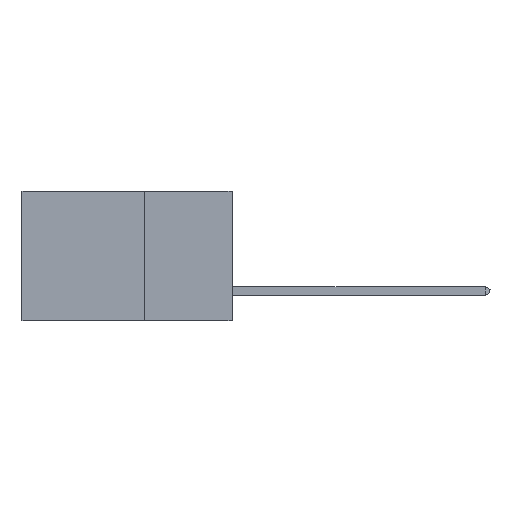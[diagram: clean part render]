
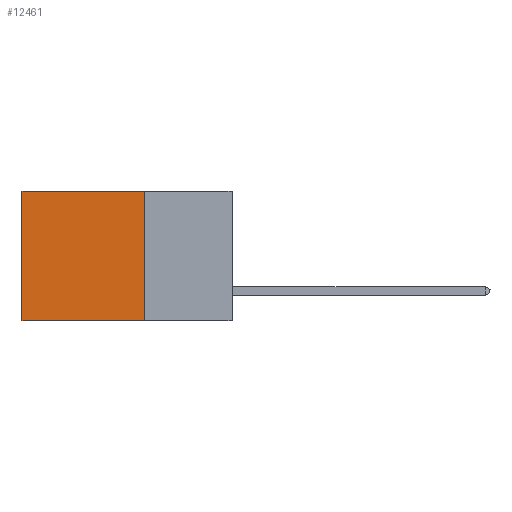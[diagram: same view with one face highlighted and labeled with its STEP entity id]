
A CAD part, left-side view. The second image highlights one B-rep face of the part: STEP entity #12461.
In plain terms, the highlighted planar face has unit normal (-1, 0, 0).
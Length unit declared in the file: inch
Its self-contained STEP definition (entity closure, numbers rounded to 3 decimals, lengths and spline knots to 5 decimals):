
#903 = EDGE_CURVE ( 'NONE', #23160, #5091, #25538, .T. ) ;
#1107 = EDGE_CURVE ( 'NONE', #5091, #11300, #23651, .T. ) ;
#1490 = DIRECTION ( 'NONE',  ( 0., 0., -1. ) ) ;
#1518 = EDGE_CURVE ( 'NONE', #23160, #22618, #10651, .T. ) ;
#2154 = CARTESIAN_POINT ( 'NONE',  ( 0.2875, 0.6, 0. ) ) ;
#5091 = VERTEX_POINT ( 'NONE', #19248 ) ;
#5260 = LINE ( 'NONE', #24532, #25609 ) ;
#5328 = VECTOR ( 'NONE', #1490, 39.37008 ) ;
#5482 = ORIENTED_EDGE ( 'NONE', *, *, #1518, .F. ) ;
#6018 = DIRECTION ( 'NONE',  ( 0., 0., -1. ) ) ;
#7809 = EDGE_CURVE ( 'NONE', #22618, #11300, #5260, .T. ) ;
#7828 = DIRECTION ( 'NONE',  ( 0., 0., -1. ) ) ;
#8459 = EDGE_LOOP ( 'NONE', ( #16489, #11627, #5482, #22404 ) ) ;
#8543 = DIRECTION ( 'NONE',  ( 0., 1., 0. ) ) ;
#9111 = PLANE ( 'NONE',  #14313 ) ;
#10651 = LINE ( 'NONE', #15129, #5328 ) ;
#11300 = VERTEX_POINT ( 'NONE', #17604 ) ;
#11627 = ORIENTED_EDGE ( 'NONE', *, *, #7809, .F. ) ;
#12461 = ADVANCED_FACE ( 'NONE', ( #14057 ), #9111, .F. ) ;
#14057 = FACE_OUTER_BOUND ( 'NONE', #8459, .T. ) ;
#14264 = VECTOR ( 'NONE', #14276, 39.37008 ) ;
#14276 = DIRECTION ( 'NONE',  ( 0., 1., 0. ) ) ;
#14313 = AXIS2_PLACEMENT_3D ( 'NONE', #17594, #23627, #7828 ) ;
#15129 = CARTESIAN_POINT ( 'NONE',  ( 0.2875, 0.25, 0. ) ) ;
#15604 = CARTESIAN_POINT ( 'NONE',  ( 0.2875, 0.25, 0. ) ) ;
#16489 = ORIENTED_EDGE ( 'NONE', *, *, #1107, .T. ) ;
#17594 = CARTESIAN_POINT ( 'NONE',  ( 0.2875, 0.25, 0. ) ) ;
#17604 = CARTESIAN_POINT ( 'NONE',  ( 0.2875, 0.6, -0.37 ) ) ;
#19248 = CARTESIAN_POINT ( 'NONE',  ( 0.2875, 0.6, 0. ) ) ;
#22391 = VECTOR ( 'NONE', #6018, 39.37008 ) ;
#22404 = ORIENTED_EDGE ( 'NONE', *, *, #903, .T. ) ;
#22618 = VERTEX_POINT ( 'NONE', #23585 ) ;
#23160 = VERTEX_POINT ( 'NONE', #15604 ) ;
#23585 = CARTESIAN_POINT ( 'NONE',  ( 0.2875, 0.25, -0.37 ) ) ;
#23627 = DIRECTION ( 'NONE',  ( 1., 0., 0. ) ) ;
#23651 = LINE ( 'NONE', #2154, #22391 ) ;
#24158 = CARTESIAN_POINT ( 'NONE',  ( 0.2875, 0.25, 0. ) ) ;
#24532 = CARTESIAN_POINT ( 'NONE',  ( 0.2875, 0.25, -0.37 ) ) ;
#25538 = LINE ( 'NONE', #24158, #14264 ) ;
#25609 = VECTOR ( 'NONE', #8543, 39.37008 ) ;
